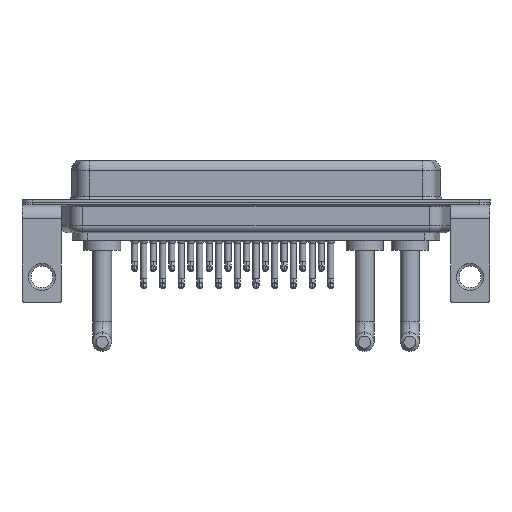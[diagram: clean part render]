
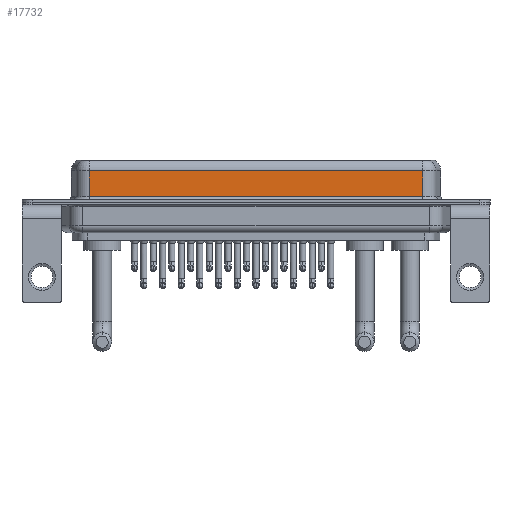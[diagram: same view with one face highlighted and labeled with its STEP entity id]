
A CAD part, front view. The second image highlights one B-rep face of the part: STEP entity #17732.
In plain terms, the highlighted planar face has unit normal (0, -1, 0).
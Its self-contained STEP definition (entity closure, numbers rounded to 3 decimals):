
#37 = FACE_OUTER_BOUND ( 'NONE', #5319, .T. ) ;
#1820 = VERTEX_POINT ( 'NONE', #16179 ) ;
#2887 = ORIENTED_EDGE ( 'NONE', *, *, #22746, .F. ) ;
#2926 = LINE ( 'NONE', #17838, #15330 ) ;
#3423 = DIRECTION ( 'NONE',  ( 0., 0., 1. ) ) ;
#3441 = ORIENTED_EDGE ( 'NONE', *, *, #9029, .T. ) ;
#5319 = EDGE_LOOP ( 'NONE', ( #2887, #20887, #9598, #3441 ) ) ;
#6571 = DIRECTION ( 'NONE',  ( -1., 0., 0. ) ) ;
#7662 = DIRECTION ( 'NONE',  ( 0., 1., 0. ) ) ;
#7903 = VERTEX_POINT ( 'NONE', #16446 ) ;
#8652 = LINE ( 'NONE', #16196, #19455 ) ;
#9029 = EDGE_CURVE ( 'NONE', #18183, #7903, #2926, .T. ) ;
#9598 = ORIENTED_EDGE ( 'NONE', *, *, #12746, .T. ) ;
#11487 = LINE ( 'NONE', #15075, #12925 ) ;
#12013 = CARTESIAN_POINT ( 'NONE',  ( 56.462, -3.95, 4.65 ) ) ;
#12533 = CARTESIAN_POINT ( 'NONE',  ( 7.038, -3.95, 0.9 ) ) ;
#12746 = EDGE_CURVE ( 'NONE', #1820, #18183, #8652, .T. ) ;
#12925 = VECTOR ( 'NONE', #19290, 1000. ) ;
#14969 = PLANE ( 'NONE',  #18817 ) ;
#15075 = CARTESIAN_POINT ( 'NONE',  ( 56.462, -3.95, 6.4 ) ) ;
#15330 = VECTOR ( 'NONE', #21915, 1000. ) ;
#15738 = CARTESIAN_POINT ( 'NONE',  ( 56.462, -3.95, 4.65 ) ) ;
#16179 = CARTESIAN_POINT ( 'NONE',  ( 7.038, -3.95, 4.65 ) ) ;
#16196 = CARTESIAN_POINT ( 'NONE',  ( 7.038, -3.95, 6.4 ) ) ;
#16446 = CARTESIAN_POINT ( 'NONE',  ( 56.462, -3.95, 0.9 ) ) ;
#17732 = ADVANCED_FACE ( 'NONE', ( #37 ), #14969, .F. ) ;
#17838 = CARTESIAN_POINT ( 'NONE',  ( 56.462, -3.95, 0.9 ) ) ;
#18183 = VERTEX_POINT ( 'NONE', #12533 ) ;
#18457 = VERTEX_POINT ( 'NONE', #12013 ) ;
#18571 = EDGE_CURVE ( 'NONE', #18457, #1820, #23543, .T. ) ;
#18817 = AXIS2_PLACEMENT_3D ( 'NONE', #22794, #7662, #3423 ) ;
#19290 = DIRECTION ( 'NONE',  ( 0., 0., -1. ) ) ;
#19455 = VECTOR ( 'NONE', #23768, 1000. ) ;
#20887 = ORIENTED_EDGE ( 'NONE', *, *, #18571, .T. ) ;
#21915 = DIRECTION ( 'NONE',  ( 1., 0., 0. ) ) ;
#22746 = EDGE_CURVE ( 'NONE', #18457, #7903, #11487, .T. ) ;
#22794 = CARTESIAN_POINT ( 'NONE',  ( 56.462, -3.95, 6.4 ) ) ;
#23543 = LINE ( 'NONE', #15738, #23591 ) ;
#23591 = VECTOR ( 'NONE', #6571, 1000. ) ;
#23768 = DIRECTION ( 'NONE',  ( 0., 0., -1. ) ) ;
